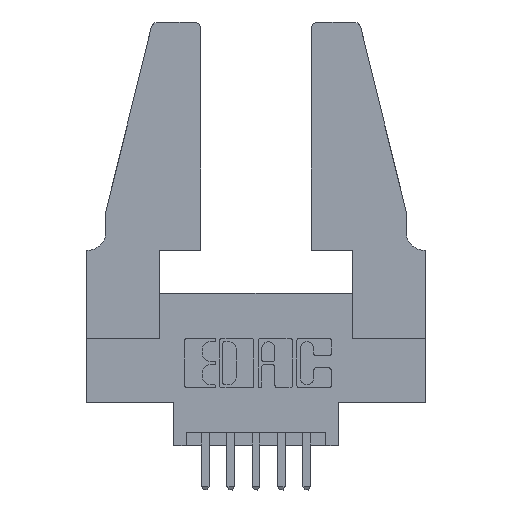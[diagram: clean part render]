
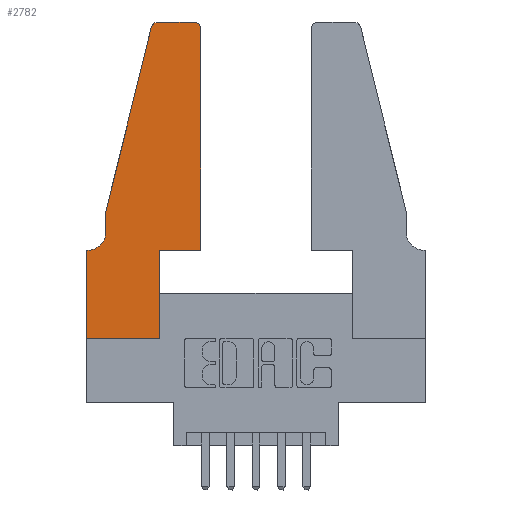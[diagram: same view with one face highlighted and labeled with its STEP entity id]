
A CAD part, top view. The second image highlights one B-rep face of the part: STEP entity #2782.
In plain terms, the highlighted planar face has unit normal (0, 0, 1).
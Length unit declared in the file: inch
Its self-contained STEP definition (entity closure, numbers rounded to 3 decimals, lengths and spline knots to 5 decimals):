
#88 = EDGE_CURVE ( 'NONE', #8121, #6124, #3290, .T. ) ;
#103 = LINE ( 'NONE', #10125, #3998 ) ;
#293 = LINE ( 'NONE', #8524, #8806 ) ;
#623 = LINE ( 'NONE', #1822, #9673 ) ;
#828 = ORIENTED_EDGE ( 'NONE', *, *, #3935, .T. ) ;
#956 = VERTEX_POINT ( 'NONE', #2936 ) ;
#1125 = ORIENTED_EDGE ( 'NONE', *, *, #5812, .T. ) ;
#1157 = ORIENTED_EDGE ( 'NONE', *, *, #1918, .T. ) ;
#1175 = VECTOR ( 'NONE', #2625, 39.37008 ) ;
#1184 = DIRECTION ( 'NONE',  ( 0., 0., 1. ) ) ;
#1209 = CARTESIAN_POINT ( 'NONE',  ( 0.0055, 0.35, 0.37 ) ) ;
#1436 = DIRECTION ( 'NONE',  ( 0., -1., 0. ) ) ;
#1557 = CIRCLE ( 'NONE', #8655, 0.03 ) ;
#1559 = ORIENTED_EDGE ( 'NONE', *, *, #7628, .T. ) ;
#1569 = VERTEX_POINT ( 'NONE', #2307 ) ;
#1656 = DIRECTION ( 'NONE',  ( 1., 0., 0. ) ) ;
#1678 = CARTESIAN_POINT ( 'NONE',  ( 0.4505, 0.35, 0.37 ) ) ;
#1723 = DIRECTION ( 'NONE',  ( 0., 1., 0. ) ) ;
#1822 = CARTESIAN_POINT ( 'NONE',  ( 0.4505, 0.35, 0.37 ) ) ;
#1828 = CIRCLE ( 'NONE', #6320, 0.03 ) ;
#1918 = EDGE_CURVE ( 'NONE', #8955, #1569, #623, .T. ) ;
#2195 = VECTOR ( 'NONE', #3338, 39.37008 ) ;
#2276 = EDGE_CURVE ( 'NONE', #956, #8899, #5840, .T. ) ;
#2307 = CARTESIAN_POINT ( 'NONE',  ( 0.4505, 1.22, 0.37 ) ) ;
#2329 = CARTESIAN_POINT ( 'NONE',  ( 0.0755, 0.5, 0.37 ) ) ;
#2625 = DIRECTION ( 'NONE',  ( -1., 0., 0. ) ) ;
#2744 = CARTESIAN_POINT ( 'NONE',  ( 0.2605, 1.25, 0.37 ) ) ;
#2782 = ADVANCED_FACE ( 'NONE', ( #3510 ), #9497, .T. ) ;
#2810 = ORIENTED_EDGE ( 'NONE', *, *, #8258, .T. ) ;
#2838 = DIRECTION ( 'NONE',  ( -1., 0., 0. ) ) ;
#2928 = EDGE_LOOP ( 'NONE', ( #9468, #6186, #8571, #1559, #7850, #828, #1125, #4172, #2810, #6207, #1157, #6294 ) ) ;
#2936 = CARTESIAN_POINT ( 'NONE',  ( 0.4205, 1.25, 0.37 ) ) ;
#3203 = CARTESIAN_POINT ( 'NONE',  ( 0., 0., 0.37 ) ) ;
#3290 = CIRCLE ( 'NONE', #4232, 0.07 ) ;
#3338 = DIRECTION ( 'NONE',  ( 0., 1., 0. ) ) ;
#3384 = CARTESIAN_POINT ( 'NONE',  ( 0.4505, 0.35, 0.37 ) ) ;
#3500 = VECTOR ( 'NONE', #9521, 39.37008 ) ;
#3510 = FACE_OUTER_BOUND ( 'NONE', #2928, .T. ) ;
#3584 = VERTEX_POINT ( 'NONE', #6446 ) ;
#3927 = DIRECTION ( 'NONE',  ( 0., 0., 1. ) ) ;
#3935 = EDGE_CURVE ( 'NONE', #6124, #5373, #8158, .T. ) ;
#3998 = VECTOR ( 'NONE', #1436, 39.37008 ) ;
#4172 = ORIENTED_EDGE ( 'NONE', *, *, #4522, .T. ) ;
#4173 = DIRECTION ( 'NONE',  ( 1., 0., 0. ) ) ;
#4232 = AXIS2_PLACEMENT_3D ( 'NONE', #6119, #5199, #2838 ) ;
#4312 = LINE ( 'NONE', #3384, #10962 ) ;
#4452 = VECTOR ( 'NONE', #11073, 39.37008 ) ;
#4472 = VERTEX_POINT ( 'NONE', #2329 ) ;
#4518 = EDGE_CURVE ( 'NONE', #8611, #4472, #7049, .T. ) ;
#4522 = EDGE_CURVE ( 'NONE', #9464, #10774, #293, .T. ) ;
#4671 = CARTESIAN_POINT ( 'NONE',  ( 0.25487, 1.22718, 0.37 ) ) ;
#5199 = DIRECTION ( 'NONE',  ( 0., 0., -1. ) ) ;
#5279 = EDGE_CURVE ( 'NONE', #3584, #8955, #4312, .T. ) ;
#5373 = VERTEX_POINT ( 'NONE', #7896 ) ;
#5475 = EDGE_CURVE ( 'NONE', #8899, #8611, #1828, .T. ) ;
#5519 = VECTOR ( 'NONE', #10368, 39.37008 ) ;
#5555 = EDGE_CURVE ( 'NONE', #1569, #956, #1557, .T. ) ;
#5812 = EDGE_CURVE ( 'NONE', #5373, #9464, #10143, .T. ) ;
#5840 = LINE ( 'NONE', #2744, #1175 ) ;
#5884 = CARTESIAN_POINT ( 'NONE',  ( 0.0755, 0.5, 0.37 ) ) ;
#5925 = AXIS2_PLACEMENT_3D ( 'NONE', #9458, #9444, #10991 ) ;
#6119 = CARTESIAN_POINT ( 'NONE',  ( 0.0055, 0.42, 0.37 ) ) ;
#6124 = VERTEX_POINT ( 'NONE', #1209 ) ;
#6186 = ORIENTED_EDGE ( 'NONE', *, *, #5475, .T. ) ;
#6207 = ORIENTED_EDGE ( 'NONE', *, *, #5279, .T. ) ;
#6294 = ORIENTED_EDGE ( 'NONE', *, *, #5555, .T. ) ;
#6320 = AXIS2_PLACEMENT_3D ( 'NONE', #6448, #1184, #7328 ) ;
#6446 = CARTESIAN_POINT ( 'NONE',  ( 0.2865, 0.35, 0.37 ) ) ;
#6448 = CARTESIAN_POINT ( 'NONE',  ( 0.284, 1.22, 0.37 ) ) ;
#7049 = LINE ( 'NONE', #5884, #4452 ) ;
#7328 = DIRECTION ( 'NONE',  ( 1., 0., 0. ) ) ;
#7628 = EDGE_CURVE ( 'NONE', #4472, #8121, #103, .T. ) ;
#7850 = ORIENTED_EDGE ( 'NONE', *, *, #88, .T. ) ;
#7896 = CARTESIAN_POINT ( 'NONE',  ( 0., 0.35, 0.37 ) ) ;
#8121 = VERTEX_POINT ( 'NONE', #9256 ) ;
#8155 = CARTESIAN_POINT ( 'NONE',  ( 0.2865, 0., 0.37 ) ) ;
#8158 = LINE ( 'NONE', #9551, #3500 ) ;
#8258 = EDGE_CURVE ( 'NONE', #10774, #3584, #9166, .T. ) ;
#8524 = CARTESIAN_POINT ( 'NONE',  ( 0., 0., 0.37 ) ) ;
#8571 = ORIENTED_EDGE ( 'NONE', *, *, #4518, .T. ) ;
#8586 = CARTESIAN_POINT ( 'NONE',  ( 0.2865, 0.35, 0.37 ) ) ;
#8611 = VERTEX_POINT ( 'NONE', #4671 ) ;
#8655 = AXIS2_PLACEMENT_3D ( 'NONE', #9130, #3927, #9989 ) ;
#8806 = VECTOR ( 'NONE', #4173, 39.37008 ) ;
#8899 = VERTEX_POINT ( 'NONE', #10319 ) ;
#8955 = VERTEX_POINT ( 'NONE', #1678 ) ;
#9130 = CARTESIAN_POINT ( 'NONE',  ( 0.4205, 1.22, 0.37 ) ) ;
#9166 = LINE ( 'NONE', #8586, #2195 ) ;
#9256 = CARTESIAN_POINT ( 'NONE',  ( 0.0755, 0.42, 0.37 ) ) ;
#9444 = DIRECTION ( 'NONE',  ( 0., 0., 1. ) ) ;
#9458 = CARTESIAN_POINT ( 'NONE',  ( 0., 0.35, 0.37 ) ) ;
#9464 = VERTEX_POINT ( 'NONE', #3203 ) ;
#9468 = ORIENTED_EDGE ( 'NONE', *, *, #2276, .T. ) ;
#9497 = PLANE ( 'NONE',  #5925 ) ;
#9521 = DIRECTION ( 'NONE',  ( -1., 0., 0. ) ) ;
#9551 = CARTESIAN_POINT ( 'NONE',  ( 0.0755, 0.35, 0.37 ) ) ;
#9673 = VECTOR ( 'NONE', #1723, 39.37008 ) ;
#9989 = DIRECTION ( 'NONE',  ( 1., 0., 0. ) ) ;
#10125 = CARTESIAN_POINT ( 'NONE',  ( 0.0755, 0.5, 0.37 ) ) ;
#10143 = LINE ( 'NONE', #11198, #5519 ) ;
#10319 = CARTESIAN_POINT ( 'NONE',  ( 0.284, 1.25, 0.37 ) ) ;
#10368 = DIRECTION ( 'NONE',  ( 0., -1., 0. ) ) ;
#10774 = VERTEX_POINT ( 'NONE', #8155 ) ;
#10962 = VECTOR ( 'NONE', #1656, 39.37008 ) ;
#10991 = DIRECTION ( 'NONE',  ( 1., 0., 0. ) ) ;
#11073 = DIRECTION ( 'NONE',  ( -0.239, -0.971, 0. ) ) ;
#11198 = CARTESIAN_POINT ( 'NONE',  ( 0., 0., 0.37 ) ) ;
